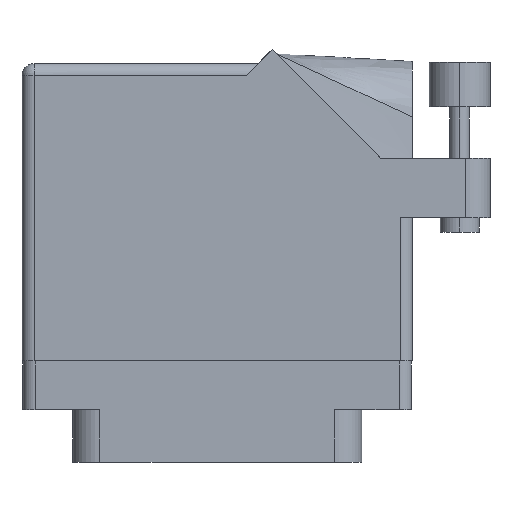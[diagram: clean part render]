
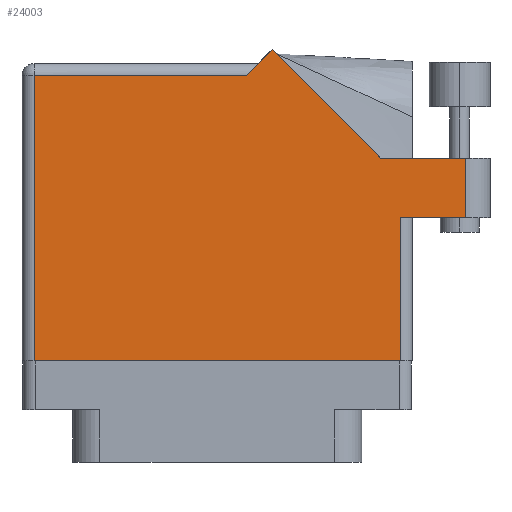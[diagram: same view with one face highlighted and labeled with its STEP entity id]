
A CAD part, front view. The second image highlights one B-rep face of the part: STEP entity #24003.
In plain terms, the highlighted face is planar.
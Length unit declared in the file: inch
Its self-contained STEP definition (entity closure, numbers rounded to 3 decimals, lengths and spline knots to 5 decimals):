
#93 = LINE ( 'NONE', #25609, #21042 ) ;
#1782 = CARTESIAN_POINT ( 'NONE',  ( 1.28, 0.944, 0.455 ) ) ;
#2394 = AXIS2_PLACEMENT_3D ( 'NONE', #13759, #19504, #5743 ) ;
#2907 = EDGE_CURVE ( 'NONE', #35936, #25068, #17759, .T. ) ;
#2934 = VERTEX_POINT ( 'NONE', #34708 ) ;
#3344 = CARTESIAN_POINT ( 'NONE',  ( 1.005, 0.637, 0.455 ) ) ;
#3655 = VERTEX_POINT ( 'NONE', #4762 ) ;
#3994 = EDGE_CURVE ( 'NONE', #5520, #3655, #20777, .T. ) ;
#4000 = DIRECTION ( 'NONE',  ( 0., -1., 0. ) ) ;
#4589 = CARTESIAN_POINT ( 'NONE',  ( 1.28, 0.637, 0.455 ) ) ;
#4762 = CARTESIAN_POINT ( 'NONE',  ( -0.943, -0.1, 0.455 ) ) ;
#5520 = VERTEX_POINT ( 'NONE', #13874 ) ;
#5563 = CARTESIAN_POINT ( 'NONE',  ( 0.943, 0.637, 0.455 ) ) ;
#5680 = ORIENTED_EDGE ( 'NONE', *, *, #29299, .T. ) ;
#5743 = DIRECTION ( 'NONE',  ( -1., 0., 0. ) ) ;
#6051 = ORIENTED_EDGE ( 'NONE', *, *, #15717, .T. ) ;
#6628 = ORIENTED_EDGE ( 'NONE', *, *, #3994, .T. ) ;
#7377 = DIRECTION ( 'NONE',  ( 0., 1., 0. ) ) ;
#7827 = LINE ( 'NONE', #14937, #28730 ) ;
#8363 = DIRECTION ( 'NONE',  ( 0., 1., 0. ) ) ;
#9168 = DIRECTION ( 'NONE',  ( 1., 0., 0. ) ) ;
#9307 = EDGE_CURVE ( 'NONE', #31459, #12032, #19797, .T. ) ;
#10336 = VECTOR ( 'NONE', #7377, 39.37008 ) ;
#10392 = VECTOR ( 'NONE', #9168, 39.37008 ) ;
#10495 = FACE_OUTER_BOUND ( 'NONE', #12323, .T. ) ;
#11220 = ORIENTED_EDGE ( 'NONE', *, *, #35895, .T. ) ;
#11245 = ORIENTED_EDGE ( 'NONE', *, *, #14070, .T. ) ;
#11255 = EDGE_CURVE ( 'NONE', #12032, #5520, #93, .T. ) ;
#11889 = VECTOR ( 'NONE', #25769, 39.37008 ) ;
#12032 = VERTEX_POINT ( 'NONE', #26208 ) ;
#12323 = EDGE_LOOP ( 'NONE', ( #30744, #11220, #34419, #6051, #30743, #25065, #6628, #11245, #5680 ) ) ;
#12340 = CARTESIAN_POINT ( 'NONE',  ( -1.005, -0.1, 0.455 ) ) ;
#13759 = CARTESIAN_POINT ( 'NONE',  ( -1.005, 1.43, 0.455 ) ) ;
#13874 = CARTESIAN_POINT ( 'NONE',  ( -0.943, 1.368, 0.455 ) ) ;
#14057 = VECTOR ( 'NONE', #8363, 39.37008 ) ;
#14070 = EDGE_CURVE ( 'NONE', #3655, #14261, #20583, .T. ) ;
#14261 = VERTEX_POINT ( 'NONE', #33651 ) ;
#14937 = CARTESIAN_POINT ( 'NONE',  ( 1.405, 0.944, 0.455 ) ) ;
#15717 = EDGE_CURVE ( 'NONE', #2934, #31459, #32902, .T. ) ;
#16379 = VECTOR ( 'NONE', #4000, 39.37008 ) ;
#17759 = LINE ( 'NONE', #3344, #10392 ) ;
#19293 = CARTESIAN_POINT ( 'NONE',  ( 0.28271, 1.50071, 0.455 ) ) ;
#19504 = DIRECTION ( 'NONE',  ( 0., 0., -1. ) ) ;
#19797 = LINE ( 'NONE', #33482, #28472 ) ;
#20379 = LINE ( 'NONE', #1782, #10336 ) ;
#20583 = LINE ( 'NONE', #12340, #34579 ) ;
#20777 = LINE ( 'NONE', #23973, #16379 ) ;
#21042 = VECTOR ( 'NONE', #28373, 39.37008 ) ;
#21528 = LINE ( 'NONE', #5563, #14057 ) ;
#21946 = DIRECTION ( 'NONE',  ( 1., 0., 0. ) ) ;
#22004 = DIRECTION ( 'NONE',  ( -0.707, -0.707, 0. ) ) ;
#22470 = VERTEX_POINT ( 'NONE', #26190 ) ;
#22831 = CARTESIAN_POINT ( 'NONE',  ( 0.83942, 0.944, 0.455 ) ) ;
#23973 = CARTESIAN_POINT ( 'NONE',  ( -0.943, -0.1, 0.455 ) ) ;
#24003 = ADVANCED_FACE ( 'NONE', ( #10495 ), #30857, .F. ) ;
#25065 = ORIENTED_EDGE ( 'NONE', *, *, #11255, .T. ) ;
#25068 = VERTEX_POINT ( 'NONE', #4589 ) ;
#25609 = CARTESIAN_POINT ( 'NONE',  ( -1.005, 1.368, 0.455 ) ) ;
#25769 = DIRECTION ( 'NONE',  ( -0.707, 0.707, 0. ) ) ;
#26190 = CARTESIAN_POINT ( 'NONE',  ( 1.28, 0.944, 0.455 ) ) ;
#26200 = DIRECTION ( 'NONE',  ( -1., 0., 0. ) ) ;
#26208 = CARTESIAN_POINT ( 'NONE',  ( 0.15, 1.368, 0.455 ) ) ;
#26878 = CARTESIAN_POINT ( 'NONE',  ( 0.943, 0.637, 0.455 ) ) ;
#28373 = DIRECTION ( 'NONE',  ( -1., 0., 0. ) ) ;
#28472 = VECTOR ( 'NONE', #22004, 39.37008 ) ;
#28730 = VECTOR ( 'NONE', #26200, 39.37008 ) ;
#29299 = EDGE_CURVE ( 'NONE', #14261, #35936, #21528, .T. ) ;
#30743 = ORIENTED_EDGE ( 'NONE', *, *, #9307, .T. ) ;
#30744 = ORIENTED_EDGE ( 'NONE', *, *, #2907, .T. ) ;
#30857 = PLANE ( 'NONE',  #2394 ) ;
#31459 = VERTEX_POINT ( 'NONE', #19293 ) ;
#31676 = EDGE_CURVE ( 'NONE', #22470, #2934, #7827, .T. ) ;
#32902 = LINE ( 'NONE', #22831, #11889 ) ;
#33482 = CARTESIAN_POINT ( 'NONE',  ( 0.212, 1.43, 0.455 ) ) ;
#33651 = CARTESIAN_POINT ( 'NONE',  ( 0.943, -0.1, 0.455 ) ) ;
#34419 = ORIENTED_EDGE ( 'NONE', *, *, #31676, .T. ) ;
#34579 = VECTOR ( 'NONE', #21946, 39.37008 ) ;
#34708 = CARTESIAN_POINT ( 'NONE',  ( 0.83942, 0.944, 0.455 ) ) ;
#35895 = EDGE_CURVE ( 'NONE', #25068, #22470, #20379, .T. ) ;
#35936 = VERTEX_POINT ( 'NONE', #26878 ) ;
